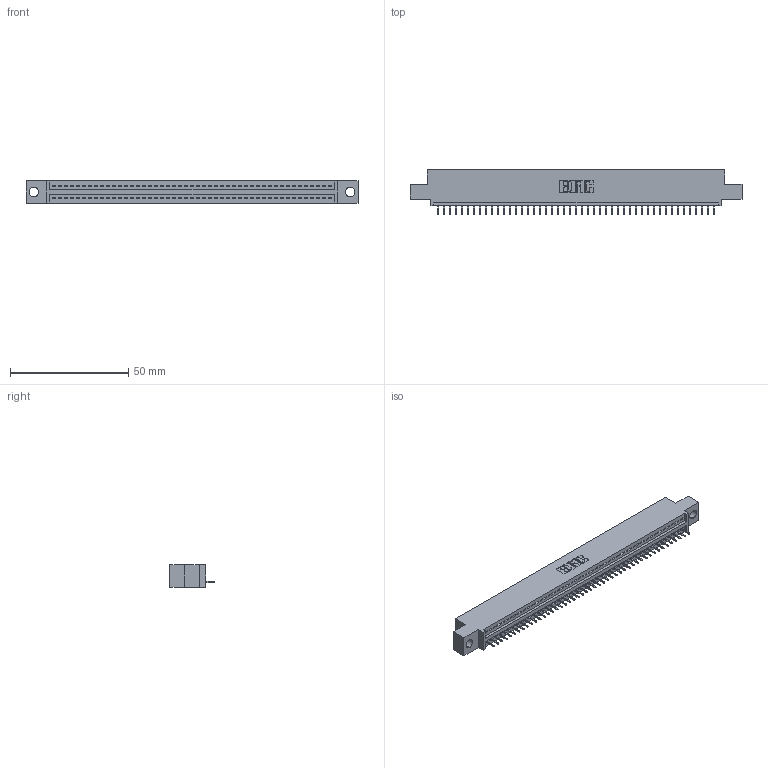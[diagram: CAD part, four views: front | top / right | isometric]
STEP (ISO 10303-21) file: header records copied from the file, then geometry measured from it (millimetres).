
FILE_DESCRIPTION (( 'STEP AP203' ), '1' );
FILE_NAME ('345-047-525-404.STEP', '2020-09-20T00:33:57', ( '' ), ( '' ), 'SwSTEP 2.0', 'SolidWorks 2020', '' );
FILE_SCHEMA (( 'CONFIG_CONTROL_DESIGN' ));
Length unit declared in the file: inch
Products named in the file (3): 345-292-001_345-293-125; 345-047-525-404; 345 Part_0.110 Offset - 0.156 Dia-TH
Assembly tree (48 placements, depth 2):
  345-047-525-404
    345 Part_0.110 Offset - 0.156 Dia-TH
    345-292-001_345-293-125  x47
Bounding box: 140.59 x 18.72 x 9.4 mm (x, y, z)
Volume: 13041.1 mm3; surface area: 16649.1 mm2
Topology: 48 solids, 48 shells, 3044 faces, 8813 edges, 5686 vertices
Faces by surface type: plane 2246, cylinder 798
Entity records: 34909 total; most frequent: CARTESIAN_POINT 6053, ORIENTED_EDGE 6034, DIRECTION 5279, EDGE_CURVE 3017, LINE 2701, VECTOR 2701, VERTEX_POINT 2006, AXIS2_PLACEMENT_3D 1289
